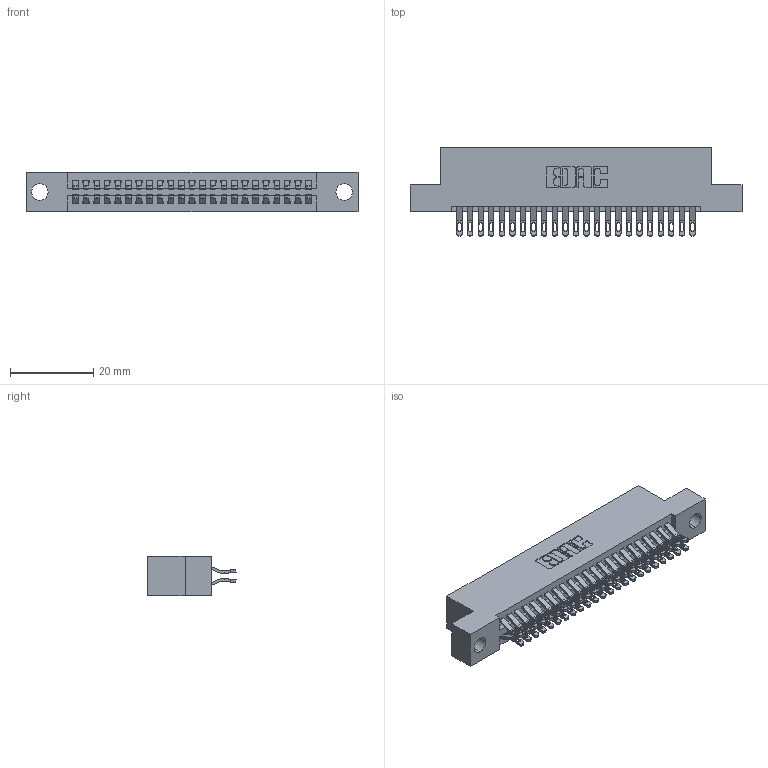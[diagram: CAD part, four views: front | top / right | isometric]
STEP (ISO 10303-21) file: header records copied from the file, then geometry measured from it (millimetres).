
FILE_DESCRIPTION (( 'STEP AP203' ), '1' );
FILE_NAME ('395-046-555-204.STEP', '2021-06-16T23:08:39', ( '' ), ( '' ), 'SwSTEP 2.0', 'SolidWorks 2020', '' );
FILE_SCHEMA (( 'CONFIG_CONTROL_DESIGN' ));
Length unit declared in the file: inch
Products named in the file (3): 395-046-555-204; 345 Part_Flush Mounting Lugs - 0.156 Dia-TI; 345-292-001_555 Tail
Assembly tree (47 placements, depth 2):
  395-046-555-204
    345 Part_Flush Mounting Lugs - 0.156 Dia-TI
    345-292-001_555 Tail  x46
Bounding box: 79.63 x 21.13 x 9.4 mm (x, y, z)
Volume: 7586.4 mm3; surface area: 11161.6 mm2
Topology: 47 solids, 47 shells, 2716 faces, 8519 edges, 5678 vertices
Faces by surface type: plane 1520, cylinder 1196
Entity records: 21349 total; most frequent: CARTESIAN_POINT 3636, ORIENTED_EDGE 3538, DIRECTION 3197, EDGE_CURVE 1769, LINE 1525, VECTOR 1525, VERTEX_POINT 1178, AXIS2_PLACEMENT_3D 836
